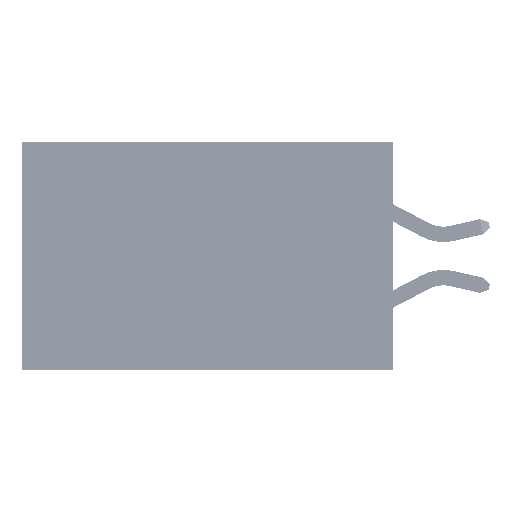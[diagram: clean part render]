
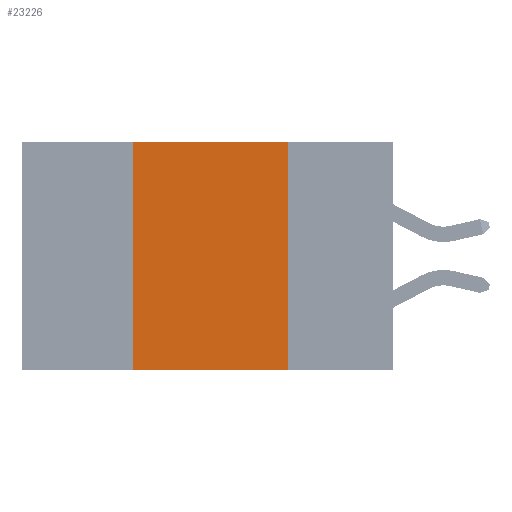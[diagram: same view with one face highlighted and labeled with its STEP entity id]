
A CAD part, left-side view. The second image highlights one B-rep face of the part: STEP entity #23226.
In plain terms, the highlighted planar face has unit normal (-1, 0, 0).
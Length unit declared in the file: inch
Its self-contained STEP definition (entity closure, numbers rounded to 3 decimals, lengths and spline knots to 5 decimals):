
#713 = EDGE_CURVE ( 'NONE', #38152, #20117, #14979, .T. ) ;
#1107 = VERTEX_POINT ( 'NONE', #41869 ) ;
#6929 = CARTESIAN_POINT ( 'NONE',  ( 0., 0.6, -0.37 ) ) ;
#8109 = CARTESIAN_POINT ( 'NONE',  ( 0., 0.42, 0. ) ) ;
#8593 = DIRECTION ( 'NONE',  ( 0., 0., 1. ) ) ;
#8932 = ORIENTED_EDGE ( 'NONE', *, *, #32545, .F. ) ;
#9006 = AXIS2_PLACEMENT_3D ( 'NONE', #36271, #20379, #12452 ) ;
#9339 = PLANE ( 'NONE',  #9006 ) ;
#10295 = VECTOR ( 'NONE', #8593, 39.37008 ) ;
#11465 = VERTEX_POINT ( 'NONE', #32469 ) ;
#12452 = DIRECTION ( 'NONE',  ( 0., 0., -1. ) ) ;
#12952 = CARTESIAN_POINT ( 'NONE',  ( 0., 0.17, 0. ) ) ;
#14979 = LINE ( 'NONE', #30618, #23301 ) ;
#16084 = ORIENTED_EDGE ( 'NONE', *, *, #43613, .T. ) ;
#20117 = VERTEX_POINT ( 'NONE', #28136 ) ;
#20379 = DIRECTION ( 'NONE',  ( 1., 0., 0. ) ) ;
#23226 = ADVANCED_FACE ( 'NONE', ( #24485 ), #9339, .F. ) ;
#23272 = ORIENTED_EDGE ( 'NONE', *, *, #713, .F. ) ;
#23301 = VECTOR ( 'NONE', #46271, 39.37008 ) ;
#24390 = EDGE_LOOP ( 'NONE', ( #33548, #23272, #8932, #16084 ) ) ;
#24485 = FACE_OUTER_BOUND ( 'NONE', #24390, .T. ) ;
#27186 = DIRECTION ( 'NONE',  ( 0., -1., 0. ) ) ;
#28136 = CARTESIAN_POINT ( 'NONE',  ( 0., 0.17, 0. ) ) ;
#28336 = LINE ( 'NONE', #8109, #10295 ) ;
#28499 = CARTESIAN_POINT ( 'NONE',  ( 0., 0.42, 0. ) ) ;
#28581 = DIRECTION ( 'NONE',  ( 0., 0., -1. ) ) ;
#30618 = CARTESIAN_POINT ( 'NONE',  ( 0., 0.6, 0. ) ) ;
#32469 = CARTESIAN_POINT ( 'NONE',  ( 0., 0.17, -0.37 ) ) ;
#32545 = EDGE_CURVE ( 'NONE', #1107, #38152, #28336, .T. ) ;
#33548 = ORIENTED_EDGE ( 'NONE', *, *, #35954, .F. ) ;
#35954 = EDGE_CURVE ( 'NONE', #20117, #11465, #48081, .T. ) ;
#36271 = CARTESIAN_POINT ( 'NONE',  ( 0., 0.6, 0. ) ) ;
#37455 = VECTOR ( 'NONE', #28581, 39.37008 ) ;
#38152 = VERTEX_POINT ( 'NONE', #28499 ) ;
#41869 = CARTESIAN_POINT ( 'NONE',  ( 0., 0.42, -0.37 ) ) ;
#42336 = LINE ( 'NONE', #6929, #47374 ) ;
#43613 = EDGE_CURVE ( 'NONE', #1107, #11465, #42336, .T. ) ;
#46271 = DIRECTION ( 'NONE',  ( 0., -1., 0. ) ) ;
#47374 = VECTOR ( 'NONE', #27186, 39.37008 ) ;
#48081 = LINE ( 'NONE', #12952, #37455 ) ;
